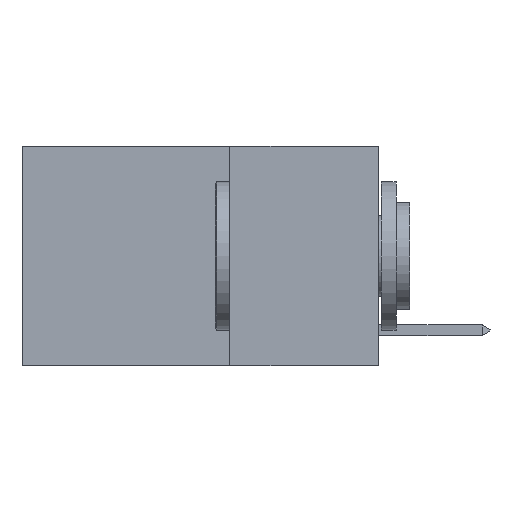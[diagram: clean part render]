
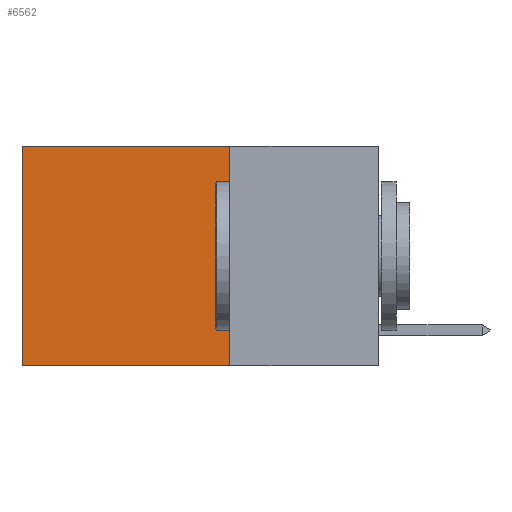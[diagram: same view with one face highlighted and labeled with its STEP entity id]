
A CAD part, left-side view. The second image highlights one B-rep face of the part: STEP entity #6562.
In plain terms, the highlighted planar face has unit normal (-1, 0, 0).
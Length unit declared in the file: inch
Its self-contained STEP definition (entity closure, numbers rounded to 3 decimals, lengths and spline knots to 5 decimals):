
#4 = VERTEX_POINT ( 'NONE', #16379 ) ;
#10 = PLANE ( 'NONE',  #9810 ) ;
#233 = VECTOR ( 'NONE', #13926, 39.37008 ) ;
#642 = LINE ( 'NONE', #12564, #4318 ) ;
#865 = CARTESIAN_POINT ( 'NONE',  ( 0.2625, 0.6, 0. ) ) ;
#2041 = CARTESIAN_POINT ( 'NONE',  ( 0.2625, 0.25, 0. ) ) ;
#2296 = VERTEX_POINT ( 'NONE', #7083 ) ;
#4318 = VECTOR ( 'NONE', #13905, 39.37008 ) ;
#4952 = VERTEX_POINT ( 'NONE', #2041 ) ;
#6159 = EDGE_CURVE ( 'NONE', #2296, #10054, #642, .T. ) ;
#6283 = LINE ( 'NONE', #865, #9309 ) ;
#6562 = ADVANCED_FACE ( 'NONE', ( #8599 ), #10, .F. ) ;
#6834 = CARTESIAN_POINT ( 'NONE',  ( 0.2625, 0.25, 0. ) ) ;
#7083 = CARTESIAN_POINT ( 'NONE',  ( 0.2625, 0.25, -0.37 ) ) ;
#7096 = ORIENTED_EDGE ( 'NONE', *, *, #15390, .T. ) ;
#7272 = ORIENTED_EDGE ( 'NONE', *, *, #6159, .F. ) ;
#7290 = ORIENTED_EDGE ( 'NONE', *, *, #11638, .F. ) ;
#7392 = CARTESIAN_POINT ( 'NONE',  ( 0.2625, 0.25, 0. ) ) ;
#7613 = ORIENTED_EDGE ( 'NONE', *, *, #12767, .T. ) ;
#7624 = VECTOR ( 'NONE', #15129, 39.37008 ) ;
#8141 = DIRECTION ( 'NONE',  ( 0., 0., -1. ) ) ;
#8599 = FACE_OUTER_BOUND ( 'NONE', #16629, .T. ) ;
#9309 = VECTOR ( 'NONE', #10164, 39.37008 ) ;
#9810 = AXIS2_PLACEMENT_3D ( 'NONE', #6834, #15960, #8141 ) ;
#10054 = VERTEX_POINT ( 'NONE', #15876 ) ;
#10164 = DIRECTION ( 'NONE',  ( 0., 0., -1. ) ) ;
#11090 = LINE ( 'NONE', #13891, #7624 ) ;
#11638 = EDGE_CURVE ( 'NONE', #4952, #2296, #13798, .T. ) ;
#12564 = CARTESIAN_POINT ( 'NONE',  ( 0.2625, 0.25, -0.37 ) ) ;
#12767 = EDGE_CURVE ( 'NONE', #4952, #4, #11090, .T. ) ;
#13798 = LINE ( 'NONE', #7392, #233 ) ;
#13891 = CARTESIAN_POINT ( 'NONE',  ( 0.2625, 0.25, 0. ) ) ;
#13905 = DIRECTION ( 'NONE',  ( 0., 1., 0. ) ) ;
#13926 = DIRECTION ( 'NONE',  ( 0., 0., -1. ) ) ;
#15129 = DIRECTION ( 'NONE',  ( 0., 1., 0. ) ) ;
#15390 = EDGE_CURVE ( 'NONE', #4, #10054, #6283, .T. ) ;
#15876 = CARTESIAN_POINT ( 'NONE',  ( 0.2625, 0.6, -0.37 ) ) ;
#15960 = DIRECTION ( 'NONE',  ( 1., 0., 0. ) ) ;
#16379 = CARTESIAN_POINT ( 'NONE',  ( 0.2625, 0.6, 0. ) ) ;
#16629 = EDGE_LOOP ( 'NONE', ( #7096, #7272, #7290, #7613 ) ) ;
